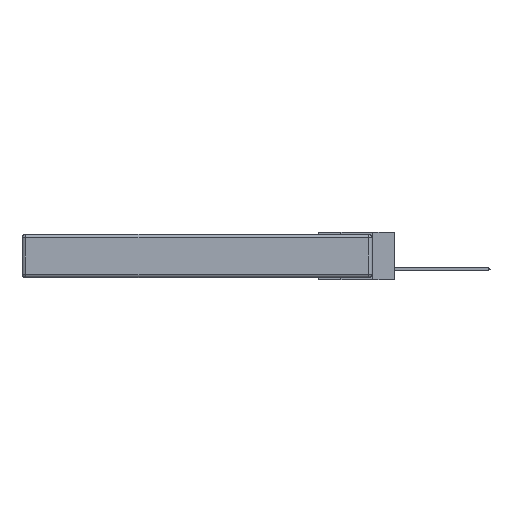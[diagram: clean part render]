
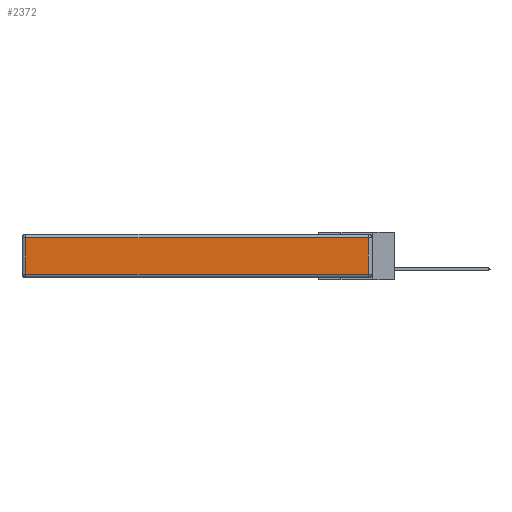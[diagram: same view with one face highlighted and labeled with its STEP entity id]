
A CAD part, left-side view. The second image highlights one B-rep face of the part: STEP entity #2372.
In plain terms, the highlighted planar face has unit normal (-1, 0, 0).
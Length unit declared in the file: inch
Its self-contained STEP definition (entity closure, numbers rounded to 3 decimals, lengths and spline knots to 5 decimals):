
#28 = VECTOR ( 'NONE', #4000, 39.37008 ) ;
#222 = DIRECTION ( 'NONE',  ( 0., 0., 1. ) ) ;
#341 = LINE ( 'NONE', #14345, #3581 ) ;
#975 = EDGE_CURVE ( 'NONE', #7155, #7994, #15329, .T. ) ;
#1130 = PLANE ( 'NONE',  #4099 ) ;
#1572 = VERTEX_POINT ( 'NONE', #3340 ) ;
#2372 = ADVANCED_FACE ( 'NONE', ( #19148 ), #1130, .T. ) ;
#3123 = EDGE_CURVE ( 'NONE', #7994, #7372, #341, .T. ) ;
#3208 = LINE ( 'NONE', #10742, #12290 ) ;
#3340 = CARTESIAN_POINT ( 'NONE',  ( 0., 2.72, -0.03 ) ) ;
#3581 = VECTOR ( 'NONE', #222, 39.37008 ) ;
#4000 = DIRECTION ( 'NONE',  ( 0., 0., -1. ) ) ;
#4099 = AXIS2_PLACEMENT_3D ( 'NONE', #13712, #18360, #15314 ) ;
#6166 = ORIENTED_EDGE ( 'NONE', *, *, #6830, .T. ) ;
#6830 = EDGE_CURVE ( 'NONE', #7372, #1572, #3208, .T. ) ;
#7155 = VERTEX_POINT ( 'NONE', #8646 ) ;
#7372 = VERTEX_POINT ( 'NONE', #20362 ) ;
#7994 = VERTEX_POINT ( 'NONE', #14258 ) ;
#8354 = ORIENTED_EDGE ( 'NONE', *, *, #16687, .T. ) ;
#8646 = CARTESIAN_POINT ( 'NONE',  ( 0., 2.72, -0.313 ) ) ;
#8934 = ORIENTED_EDGE ( 'NONE', *, *, #3123, .T. ) ;
#10742 = CARTESIAN_POINT ( 'NONE',  ( 0., 2.75, -0.03 ) ) ;
#11611 = CARTESIAN_POINT ( 'NONE',  ( 0., 0., -0.313 ) ) ;
#12290 = VECTOR ( 'NONE', #13530, 39.37008 ) ;
#13169 = DIRECTION ( 'NONE',  ( 0., -1., 0. ) ) ;
#13413 = CARTESIAN_POINT ( 'NONE',  ( 0., 2.72, -0.343 ) ) ;
#13530 = DIRECTION ( 'NONE',  ( 0., 1., 0. ) ) ;
#13712 = CARTESIAN_POINT ( 'NONE',  ( 0., 0., -0.343 ) ) ;
#14258 = CARTESIAN_POINT ( 'NONE',  ( 0., 0.03, -0.313 ) ) ;
#14345 = CARTESIAN_POINT ( 'NONE',  ( 0., 0.03, -0.343 ) ) ;
#14581 = LINE ( 'NONE', #13413, #28 ) ;
#15314 = DIRECTION ( 'NONE',  ( 0., 0., 1. ) ) ;
#15329 = LINE ( 'NONE', #11611, #19039 ) ;
#16687 = EDGE_CURVE ( 'NONE', #1572, #7155, #14581, .T. ) ;
#17557 = EDGE_LOOP ( 'NONE', ( #20441, #8934, #6166, #8354 ) ) ;
#18360 = DIRECTION ( 'NONE',  ( -1., 0., 0. ) ) ;
#19039 = VECTOR ( 'NONE', #13169, 39.37008 ) ;
#19148 = FACE_OUTER_BOUND ( 'NONE', #17557, .T. ) ;
#20362 = CARTESIAN_POINT ( 'NONE',  ( 0., 0.03, -0.03 ) ) ;
#20441 = ORIENTED_EDGE ( 'NONE', *, *, #975, .T. ) ;
